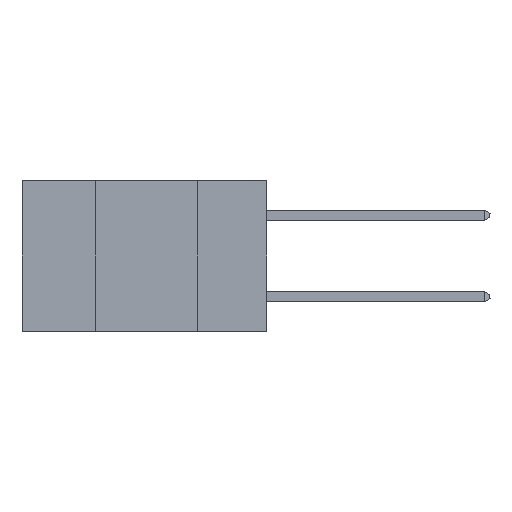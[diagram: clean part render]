
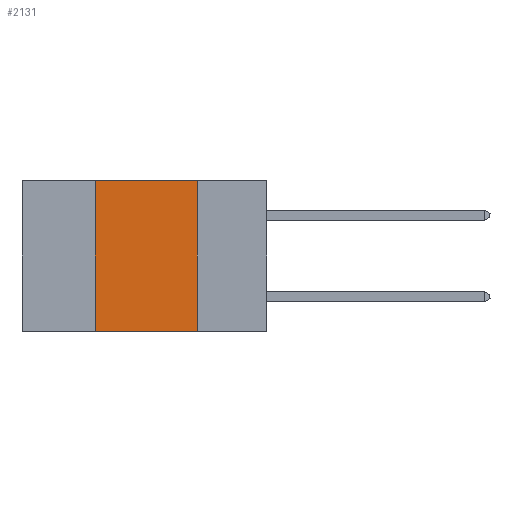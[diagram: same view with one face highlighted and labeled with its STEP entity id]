
A CAD part, left-side view. The second image highlights one B-rep face of the part: STEP entity #2131.
In plain terms, the highlighted planar face has unit normal (-1, 0, 0).
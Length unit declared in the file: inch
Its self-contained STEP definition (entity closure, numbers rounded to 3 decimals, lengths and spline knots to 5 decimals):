
#181 = CARTESIAN_POINT ( 'NONE',  ( 0., 0.42, 0. ) ) ;
#905 = ORIENTED_EDGE ( 'NONE', *, *, #28958, .F. ) ;
#2131 = ADVANCED_FACE ( 'NONE', ( #7667 ), #24399, .F. ) ;
#3077 = EDGE_CURVE ( 'NONE', #33184, #28979, #28367, .T. ) ;
#3154 = LINE ( 'NONE', #5054, #11976 ) ;
#5054 = CARTESIAN_POINT ( 'NONE',  ( 0., 0.6, -0.37 ) ) ;
#5342 = EDGE_LOOP ( 'NONE', ( #20302, #18325, #905, #20706 ) ) ;
#6380 = VECTOR ( 'NONE', #16693, 39.37008 ) ;
#6829 = DIRECTION ( 'NONE',  ( 0., -1., 0. ) ) ;
#7667 = FACE_OUTER_BOUND ( 'NONE', #5342, .T. ) ;
#7977 = CARTESIAN_POINT ( 'NONE',  ( 0., 0.6, 0. ) ) ;
#8211 = DIRECTION ( 'NONE',  ( 1., 0., 0. ) ) ;
#10769 = LINE ( 'NONE', #12124, #22201 ) ;
#10992 = VECTOR ( 'NONE', #26325, 39.37008 ) ;
#11976 = VECTOR ( 'NONE', #24305, 39.37008 ) ;
#12124 = CARTESIAN_POINT ( 'NONE',  ( 0., 0.6, 0. ) ) ;
#12191 = CARTESIAN_POINT ( 'NONE',  ( 0., 0.42, -0.37 ) ) ;
#15214 = VERTEX_POINT ( 'NONE', #12191 ) ;
#15560 = CARTESIAN_POINT ( 'NONE',  ( 0., 0.17, -0.37 ) ) ;
#16143 = CARTESIAN_POINT ( 'NONE',  ( 0., 0.17, 0. ) ) ;
#16693 = DIRECTION ( 'NONE',  ( 0., 0., -1. ) ) ;
#18325 = ORIENTED_EDGE ( 'NONE', *, *, #26338, .F. ) ;
#20302 = ORIENTED_EDGE ( 'NONE', *, *, #3077, .F. ) ;
#20706 = ORIENTED_EDGE ( 'NONE', *, *, #33205, .T. ) ;
#21453 = DIRECTION ( 'NONE',  ( 0., 0., -1. ) ) ;
#22201 = VECTOR ( 'NONE', #6829, 39.37008 ) ;
#24305 = DIRECTION ( 'NONE',  ( 0., -1., 0. ) ) ;
#24399 = PLANE ( 'NONE',  #26792 ) ;
#24734 = CARTESIAN_POINT ( 'NONE',  ( 0., 0.17, 0. ) ) ;
#25306 = VERTEX_POINT ( 'NONE', #181 ) ;
#26325 = DIRECTION ( 'NONE',  ( 0., 0., 1. ) ) ;
#26338 = EDGE_CURVE ( 'NONE', #25306, #33184, #10769, .T. ) ;
#26792 = AXIS2_PLACEMENT_3D ( 'NONE', #7977, #8211, #21453 ) ;
#28367 = LINE ( 'NONE', #24734, #6380 ) ;
#28958 = EDGE_CURVE ( 'NONE', #15214, #25306, #33388, .T. ) ;
#28979 = VERTEX_POINT ( 'NONE', #15560 ) ;
#29039 = CARTESIAN_POINT ( 'NONE',  ( 0., 0.42, 0. ) ) ;
#33184 = VERTEX_POINT ( 'NONE', #16143 ) ;
#33205 = EDGE_CURVE ( 'NONE', #15214, #28979, #3154, .T. ) ;
#33388 = LINE ( 'NONE', #29039, #10992 ) ;
